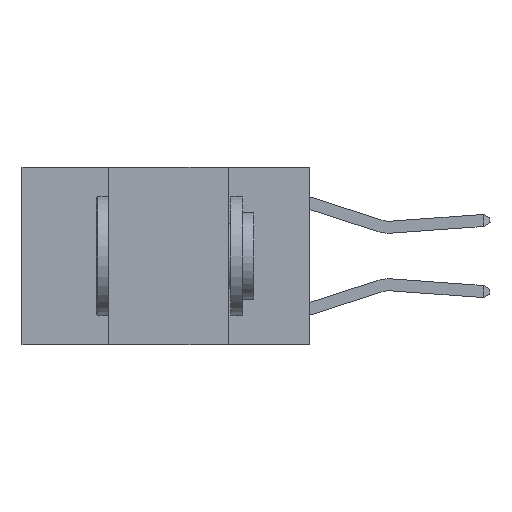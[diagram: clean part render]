
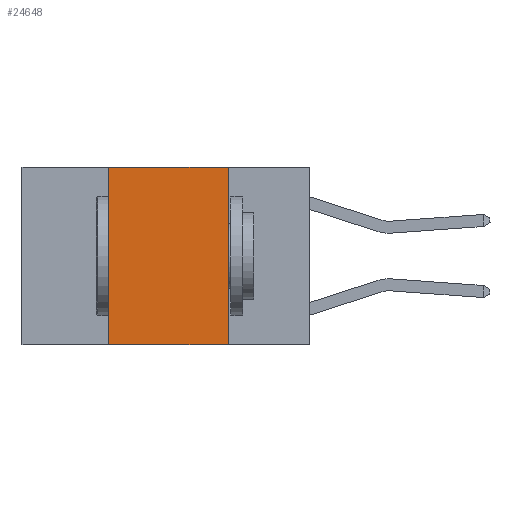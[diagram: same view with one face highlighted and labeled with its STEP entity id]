
A CAD part, left-side view. The second image highlights one B-rep face of the part: STEP entity #24648.
In plain terms, the highlighted planar face has unit normal (-1, 0, 0).
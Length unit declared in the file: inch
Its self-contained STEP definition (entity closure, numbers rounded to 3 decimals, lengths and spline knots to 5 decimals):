
#2346 = CARTESIAN_POINT ( 'NONE',  ( 0., 0.17, -0.37 ) ) ;
#3012 = ORIENTED_EDGE ( 'NONE', *, *, #13640, .F. ) ;
#3405 = VERTEX_POINT ( 'NONE', #10131 ) ;
#4176 = LINE ( 'NONE', #21812, #12123 ) ;
#5184 = ORIENTED_EDGE ( 'NONE', *, *, #14825, .T. ) ;
#5487 = CARTESIAN_POINT ( 'NONE',  ( 0., 0.6, -0.37 ) ) ;
#6350 = VECTOR ( 'NONE', #15392, 39.37008 ) ;
#7313 = LINE ( 'NONE', #23401, #13644 ) ;
#7316 = VERTEX_POINT ( 'NONE', #2346 ) ;
#7445 = AXIS2_PLACEMENT_3D ( 'NONE', #13398, #21324, #25337 ) ;
#9441 = CARTESIAN_POINT ( 'NONE',  ( 0., 0.17, 0. ) ) ;
#9512 = PLANE ( 'NONE',  #7445 ) ;
#10131 = CARTESIAN_POINT ( 'NONE',  ( 0., 0.42, 0. ) ) ;
#10261 = DIRECTION ( 'NONE',  ( 0., -1., 0. ) ) ;
#11449 = EDGE_LOOP ( 'NONE', ( #3012, #25210, #22629, #5184 ) ) ;
#12123 = VECTOR ( 'NONE', #10261, 39.37008 ) ;
#13398 = CARTESIAN_POINT ( 'NONE',  ( 0., 0.6, 0. ) ) ;
#13640 = EDGE_CURVE ( 'NONE', #15585, #7316, #15651, .T. ) ;
#13644 = VECTOR ( 'NONE', #25212, 39.37008 ) ;
#14825 = EDGE_CURVE ( 'NONE', #23595, #7316, #23633, .T. ) ;
#14939 = EDGE_CURVE ( 'NONE', #3405, #15585, #4176, .T. ) ;
#15392 = DIRECTION ( 'NONE',  ( 0., 0., -1. ) ) ;
#15585 = VERTEX_POINT ( 'NONE', #22436 ) ;
#15651 = LINE ( 'NONE', #9441, #6350 ) ;
#15666 = CARTESIAN_POINT ( 'NONE',  ( 0., 0.42, -0.37 ) ) ;
#17912 = EDGE_CURVE ( 'NONE', #23595, #3405, #7313, .T. ) ;
#19596 = VECTOR ( 'NONE', #21321, 39.37008 ) ;
#21321 = DIRECTION ( 'NONE',  ( 0., -1., 0. ) ) ;
#21324 = DIRECTION ( 'NONE',  ( 1., 0., 0. ) ) ;
#21812 = CARTESIAN_POINT ( 'NONE',  ( 0., 0.6, 0. ) ) ;
#22436 = CARTESIAN_POINT ( 'NONE',  ( 0., 0.17, 0. ) ) ;
#22629 = ORIENTED_EDGE ( 'NONE', *, *, #17912, .F. ) ;
#23269 = FACE_OUTER_BOUND ( 'NONE', #11449, .T. ) ;
#23401 = CARTESIAN_POINT ( 'NONE',  ( 0., 0.42, 0. ) ) ;
#23595 = VERTEX_POINT ( 'NONE', #15666 ) ;
#23633 = LINE ( 'NONE', #5487, #19596 ) ;
#24648 = ADVANCED_FACE ( 'NONE', ( #23269 ), #9512, .F. ) ;
#25210 = ORIENTED_EDGE ( 'NONE', *, *, #14939, .F. ) ;
#25212 = DIRECTION ( 'NONE',  ( 0., 0., 1. ) ) ;
#25337 = DIRECTION ( 'NONE',  ( 0., 0., -1. ) ) ;
